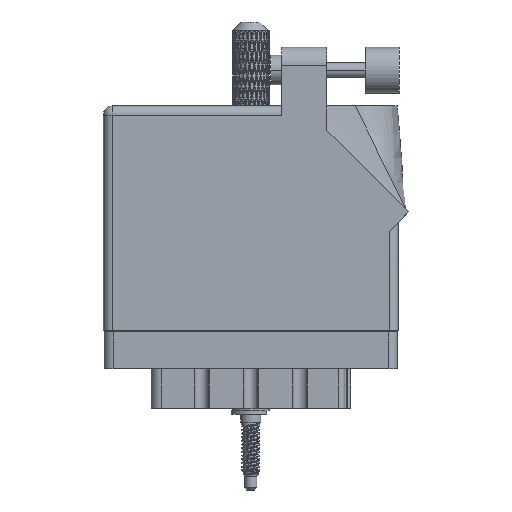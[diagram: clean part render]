
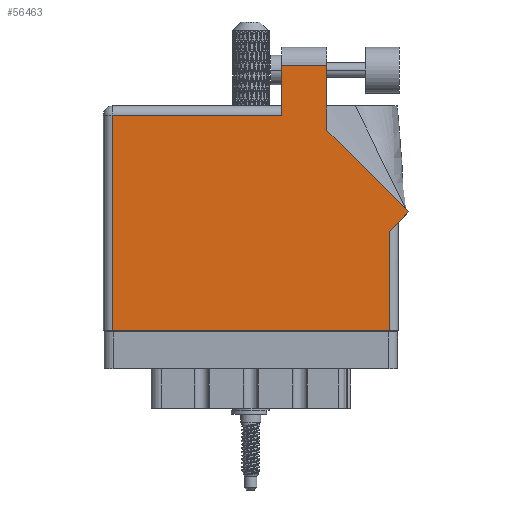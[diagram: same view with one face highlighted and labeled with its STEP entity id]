
A CAD part, front view. The second image highlights one B-rep face of the part: STEP entity #56463.
In plain terms, the highlighted face is planar.
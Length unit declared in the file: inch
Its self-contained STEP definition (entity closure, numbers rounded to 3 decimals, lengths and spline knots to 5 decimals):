
#404 = PLANE ( 'NONE',  #74583 ) ;
#1611 = ORIENTED_EDGE ( 'NONE', *, *, #57970, .T. ) ;
#2820 = EDGE_CURVE ( 'NONE', #83618, #87274, #94505, .T. ) ;
#3756 = DIRECTION ( 'NONE',  ( 0., -1., 0. ) ) ;
#6119 = CARTESIAN_POINT ( 'NONE',  ( 2.08071, 0.80771, 0. ) ) ;
#7251 = VECTOR ( 'NONE', #3756, 39.37008 ) ;
#11167 = EDGE_CURVE ( 'NONE', #70485, #83618, #80540, .T. ) ;
#11798 = CARTESIAN_POINT ( 'NONE',  ( 1.217, 1.805, 0. ) ) ;
#14903 = CARTESIAN_POINT ( 'NONE',  ( 2.08071, 0.80771, 0. ) ) ;
#16623 = FACE_OUTER_BOUND ( 'NONE', #37254, .T. ) ;
#17142 = DIRECTION ( 'NONE',  ( 0., 1., 0. ) ) ;
#21649 = LINE ( 'NONE', #34647, #44034 ) ;
#23538 = DIRECTION ( 'NONE',  ( 0., 1., 0. ) ) ;
#23618 = EDGE_CURVE ( 'NONE', #26866, #94302, #97841, .T. ) ;
#26327 = CARTESIAN_POINT ( 'NONE',  ( 2.01, 0.737, 0. ) ) ;
#26866 = VERTEX_POINT ( 'NONE', #42458 ) ;
#27486 = CARTESIAN_POINT ( 'NONE',  ( 1.217, 1.53, 0. ) ) ;
#27866 = EDGE_CURVE ( 'NONE', #94302, #70485, #78767, .T. ) ;
#28534 = CARTESIAN_POINT ( 'NONE',  ( 0.062, 1.468, 0. ) ) ;
#30384 = CARTESIAN_POINT ( 'NONE',  ( 1.524, 1.805, 0. ) ) ;
#31799 = DIRECTION ( 'NONE',  ( -1., 0., 0. ) ) ;
#34647 = CARTESIAN_POINT ( 'NONE',  ( 0., 1.468, 0. ) ) ;
#36927 = CARTESIAN_POINT ( 'NONE',  ( 1.948, 0., 0. ) ) ;
#37254 = EDGE_LOOP ( 'NONE', ( #82722, #77810, #100892, #71545, #38268, #77473, #1611, #53328, #90002 ) ) ;
#37264 = CARTESIAN_POINT ( 'NONE',  ( 1.524, 1.36442, 0. ) ) ;
#37561 = DIRECTION ( 'NONE',  ( -0.707, 0.707, 0. ) ) ;
#38268 = ORIENTED_EDGE ( 'NONE', *, *, #95724, .T. ) ;
#42458 = CARTESIAN_POINT ( 'NONE',  ( 1.948, 0.675, 0. ) ) ;
#44034 = VECTOR ( 'NONE', #59577, 39.37008 ) ;
#46283 = VECTOR ( 'NONE', #23538, 39.37008 ) ;
#46954 = VECTOR ( 'NONE', #50133, 39.37008 ) ;
#48096 = CARTESIAN_POINT ( 'NONE',  ( 0., 1.53, 0. ) ) ;
#49619 = DIRECTION ( 'NONE',  ( 0.707, 0.707, 0. ) ) ;
#50133 = DIRECTION ( 'NONE',  ( 1., 0., 0. ) ) ;
#51612 = CARTESIAN_POINT ( 'NONE',  ( 1.217, 1.805, 0. ) ) ;
#51897 = VECTOR ( 'NONE', #17142, 39.37008 ) ;
#53328 = ORIENTED_EDGE ( 'NONE', *, *, #23618, .T. ) ;
#55606 = CARTESIAN_POINT ( 'NONE',  ( 1.217, 1.468, 0. ) ) ;
#56092 = DIRECTION ( 'NONE',  ( 0., 0., -1. ) ) ;
#56463 = ADVANCED_FACE ( 'NONE', ( #16623 ), #404, .F. ) ;
#57587 = VECTOR ( 'NONE', #37561, 39.37008 ) ;
#57970 = EDGE_CURVE ( 'NONE', #80037, #26866, #89791, .T. ) ;
#59577 = DIRECTION ( 'NONE',  ( -1., 0., 0. ) ) ;
#66724 = DIRECTION ( 'NONE',  ( -1., 0., 0. ) ) ;
#68057 = LINE ( 'NONE', #95711, #46954 ) ;
#70485 = VERTEX_POINT ( 'NONE', #37264 ) ;
#71111 = VECTOR ( 'NONE', #87269, 39.37008 ) ;
#71382 = EDGE_CURVE ( 'NONE', #76885, #84019, #21649, .T. ) ;
#71545 = ORIENTED_EDGE ( 'NONE', *, *, #71382, .T. ) ;
#74200 = VECTOR ( 'NONE', #49619, 39.37008 ) ;
#74583 = AXIS2_PLACEMENT_3D ( 'NONE', #48096, #56092, #31799 ) ;
#75732 = LINE ( 'NONE', #27486, #7251 ) ;
#76885 = VERTEX_POINT ( 'NONE', #55606 ) ;
#77473 = ORIENTED_EDGE ( 'NONE', *, *, #87532, .T. ) ;
#77810 = ORIENTED_EDGE ( 'NONE', *, *, #2820, .T. ) ;
#78767 = LINE ( 'NONE', #6119, #57587 ) ;
#80037 = VERTEX_POINT ( 'NONE', #36927 ) ;
#80410 = CARTESIAN_POINT ( 'NONE',  ( 1.524, 1.36442, 0. ) ) ;
#80540 = LINE ( 'NONE', #80410, #51897 ) ;
#82722 = ORIENTED_EDGE ( 'NONE', *, *, #11167, .T. ) ;
#83618 = VERTEX_POINT ( 'NONE', #30384 ) ;
#84019 = VERTEX_POINT ( 'NONE', #28534 ) ;
#87269 = DIRECTION ( 'NONE',  ( 0., -1., 0. ) ) ;
#87274 = VERTEX_POINT ( 'NONE', #51612 ) ;
#87415 = VERTEX_POINT ( 'NONE', #95038 ) ;
#87532 = EDGE_CURVE ( 'NONE', #87415, #80037, #68057, .T. ) ;
#89791 = LINE ( 'NONE', #103132, #46283 ) ;
#90002 = ORIENTED_EDGE ( 'NONE', *, *, #27866, .T. ) ;
#92305 = LINE ( 'NONE', #95888, #71111 ) ;
#94302 = VERTEX_POINT ( 'NONE', #14903 ) ;
#94505 = LINE ( 'NONE', #11798, #97068 ) ;
#95038 = CARTESIAN_POINT ( 'NONE',  ( 0.062, 0., 0. ) ) ;
#95167 = EDGE_CURVE ( 'NONE', #87274, #76885, #75732, .T. ) ;
#95711 = CARTESIAN_POINT ( 'NONE',  ( 0., 0., 0. ) ) ;
#95724 = EDGE_CURVE ( 'NONE', #84019, #87415, #92305, .T. ) ;
#95888 = CARTESIAN_POINT ( 'NONE',  ( 0.062, 0., 0. ) ) ;
#97068 = VECTOR ( 'NONE', #66724, 39.37008 ) ;
#97841 = LINE ( 'NONE', #26327, #74200 ) ;
#100892 = ORIENTED_EDGE ( 'NONE', *, *, #95167, .T. ) ;
#103132 = CARTESIAN_POINT ( 'NONE',  ( 1.948, 0.737, 0. ) ) ;
